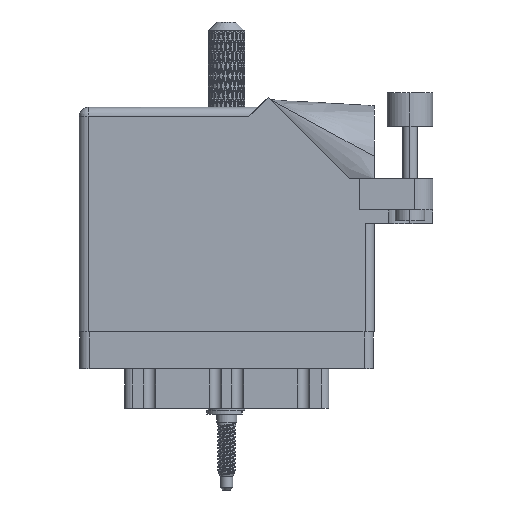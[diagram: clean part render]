
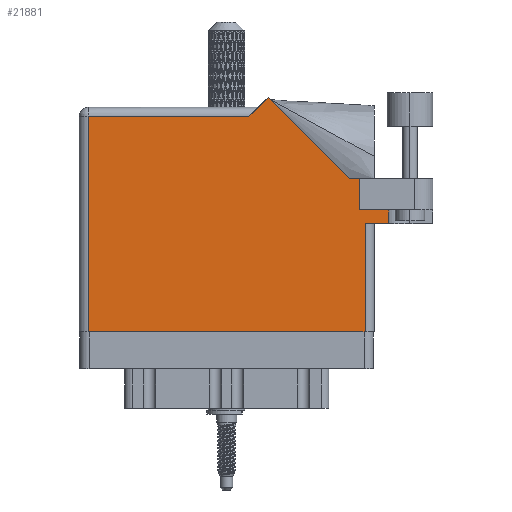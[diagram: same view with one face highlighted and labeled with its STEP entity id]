
A CAD part, front view. The second image highlights one B-rep face of the part: STEP entity #21881.
In plain terms, the highlighted face is planar.
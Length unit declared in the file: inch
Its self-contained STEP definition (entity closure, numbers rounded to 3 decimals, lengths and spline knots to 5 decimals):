
#1351 = EDGE_CURVE ( 'NONE', #46927, #65211, #44164, .T. ) ;
#1875 = VECTOR ( 'NONE', #19113, 39.37008 ) ;
#2982 = CARTESIAN_POINT ( 'NONE',  ( 1.28771, 1.60071, 0. ) ) ;
#3414 = EDGE_LOOP ( 'NONE', ( #64431, #32569, #68061, #83968, #47635, #10226, #4065, #5645, #94871, #12077, #34777 ) ) ;
#4065 = ORIENTED_EDGE ( 'NONE', *, *, #64842, .T. ) ;
#5645 = ORIENTED_EDGE ( 'NONE', *, *, #1351, .T. ) ;
#7933 = CARTESIAN_POINT ( 'NONE',  ( 2.1115, 0.737, 0. ) ) ;
#10226 = ORIENTED_EDGE ( 'NONE', *, *, #88782, .T. ) ;
#11178 = CARTESIAN_POINT ( 'NONE',  ( 1.91, 0.831, 0. ) ) ;
#12077 = ORIENTED_EDGE ( 'NONE', *, *, #70490, .T. ) ;
#12304 = VERTEX_POINT ( 'NONE', #50755 ) ;
#13783 = EDGE_CURVE ( 'NONE', #12304, #98223, #96820, .T. ) ;
#14642 = VECTOR ( 'NONE', #85014, 39.37008 ) ;
#17696 = EDGE_CURVE ( 'NONE', #98223, #33004, #19622, .T. ) ;
#19105 = VECTOR ( 'NONE', #43100, 39.37008 ) ;
#19113 = DIRECTION ( 'NONE',  ( 0., 1., 0. ) ) ;
#19622 = LINE ( 'NONE', #51916, #31186 ) ;
#19703 = CARTESIAN_POINT ( 'NONE',  ( 1.84442, 1.044, 0. ) ) ;
#20143 = DIRECTION ( 'NONE',  ( 0., -1., 0. ) ) ;
#20604 = CARTESIAN_POINT ( 'NONE',  ( 0.062, 0., 0. ) ) ;
#21535 = DIRECTION ( 'NONE',  ( -1., 0., 0. ) ) ;
#21881 = ADVANCED_FACE ( 'NONE', ( #37422 ), #69792, .F. ) ;
#24416 = VERTEX_POINT ( 'NONE', #57807 ) ;
#27063 = CARTESIAN_POINT ( 'NONE',  ( 0.062, 1.468, 0. ) ) ;
#29974 = DIRECTION ( 'NONE',  ( 0., 0., -1. ) ) ;
#31186 = VECTOR ( 'NONE', #20143, 39.37008 ) ;
#32569 = ORIENTED_EDGE ( 'NONE', *, *, #78292, .T. ) ;
#33004 = VERTEX_POINT ( 'NONE', #7933 ) ;
#33863 = VERTEX_POINT ( 'NONE', #51562 ) ;
#34357 = EDGE_CURVE ( 'NONE', #48647, #24416, #101630, .T. ) ;
#34777 = ORIENTED_EDGE ( 'NONE', *, *, #75810, .T. ) ;
#35055 = VECTOR ( 'NONE', #21535, 39.37008 ) ;
#36247 = CARTESIAN_POINT ( 'NONE',  ( 1.84442, 1.044, 0. ) ) ;
#37336 = AXIS2_PLACEMENT_3D ( 'NONE', #70317, #29974, #94724 ) ;
#37422 = FACE_OUTER_BOUND ( 'NONE', #3414, .T. ) ;
#40567 = VECTOR ( 'NONE', #48466, 39.37008 ) ;
#41432 = CARTESIAN_POINT ( 'NONE',  ( 2.01, 0.737, 0. ) ) ;
#43100 = DIRECTION ( 'NONE',  ( -0.707, 0.707, 0. ) ) ;
#43742 = CARTESIAN_POINT ( 'NONE',  ( 0., 0., 0. ) ) ;
#44164 = LINE ( 'NONE', #36247, #19105 ) ;
#45080 = DIRECTION ( 'NONE',  ( -0.707, -0.707, 0. ) ) ;
#46927 = VERTEX_POINT ( 'NONE', #19703 ) ;
#47635 = ORIENTED_EDGE ( 'NONE', *, *, #13783, .F. ) ;
#48466 = DIRECTION ( 'NONE',  ( 1., 0., 0. ) ) ;
#48647 = VERTEX_POINT ( 'NONE', #20604 ) ;
#48860 = DIRECTION ( 'NONE',  ( 1., 0., 0. ) ) ;
#49575 = CARTESIAN_POINT ( 'NONE',  ( 1.91, 1.044, 0. ) ) ;
#50669 = EDGE_CURVE ( 'NONE', #65211, #96211, #70080, .T. ) ;
#50755 = CARTESIAN_POINT ( 'NONE',  ( 1.91, 0.831, 0. ) ) ;
#51562 = CARTESIAN_POINT ( 'NONE',  ( 1.948, 0.737, 0. ) ) ;
#51916 = CARTESIAN_POINT ( 'NONE',  ( 2.1115, 1.16177, 0. ) ) ;
#53739 = DIRECTION ( 'NONE',  ( 0., 1., 0. ) ) ;
#54632 = CARTESIAN_POINT ( 'NONE',  ( 1.217, 1.53, 0. ) ) ;
#56406 = VECTOR ( 'NONE', #76155, 39.37008 ) ;
#56894 = VECTOR ( 'NONE', #82562, 39.37008 ) ;
#57807 = CARTESIAN_POINT ( 'NONE',  ( 1.948, 0., 0. ) ) ;
#58692 = VECTOR ( 'NONE', #53739, 39.37008 ) ;
#59422 = VECTOR ( 'NONE', #48860, 39.37008 ) ;
#59545 = LINE ( 'NONE', #86045, #14642 ) ;
#61194 = CARTESIAN_POINT ( 'NONE',  ( 1.948, 0.737, 0. ) ) ;
#61818 = LINE ( 'NONE', #94199, #35055 ) ;
#63855 = VERTEX_POINT ( 'NONE', #27063 ) ;
#64431 = ORIENTED_EDGE ( 'NONE', *, *, #34357, .T. ) ;
#64842 = EDGE_CURVE ( 'NONE', #103324, #46927, #59545, .T. ) ;
#65211 = VERTEX_POINT ( 'NONE', #2982 ) ;
#67151 = CARTESIAN_POINT ( 'NONE',  ( 2.1115, 0.831, 0. ) ) ;
#68061 = ORIENTED_EDGE ( 'NONE', *, *, #93259, .T. ) ;
#69172 = LINE ( 'NONE', #61194, #58692 ) ;
#69194 = VECTOR ( 'NONE', #45080, 39.37008 ) ;
#69792 = PLANE ( 'NONE',  #37336 ) ;
#70080 = LINE ( 'NONE', #54632, #69194 ) ;
#70317 = CARTESIAN_POINT ( 'NONE',  ( 0., 1.53, 0. ) ) ;
#70490 = EDGE_CURVE ( 'NONE', #96211, #63855, #61818, .T. ) ;
#71754 = LINE ( 'NONE', #41432, #59422 ) ;
#75810 = EDGE_CURVE ( 'NONE', #63855, #48647, #76179, .T. ) ;
#75852 = LINE ( 'NONE', #11178, #1875 ) ;
#76155 = DIRECTION ( 'NONE',  ( 1., 0., 0. ) ) ;
#76179 = LINE ( 'NONE', #83098, #56894 ) ;
#78292 = EDGE_CURVE ( 'NONE', #24416, #33863, #69172, .T. ) ;
#82562 = DIRECTION ( 'NONE',  ( 0., -1., 0. ) ) ;
#83098 = CARTESIAN_POINT ( 'NONE',  ( 0.062, 0., 0. ) ) ;
#83968 = ORIENTED_EDGE ( 'NONE', *, *, #17696, .F. ) ;
#85014 = DIRECTION ( 'NONE',  ( -1., 0., 0. ) ) ;
#86045 = CARTESIAN_POINT ( 'NONE',  ( 2.41, 1.044, 0. ) ) ;
#88782 = EDGE_CURVE ( 'NONE', #12304, #103324, #75852, .T. ) ;
#93259 = EDGE_CURVE ( 'NONE', #33863, #33004, #71754, .T. ) ;
#94199 = CARTESIAN_POINT ( 'NONE',  ( 0., 1.468, 0. ) ) ;
#94724 = DIRECTION ( 'NONE',  ( -1., 0., 0. ) ) ;
#94871 = ORIENTED_EDGE ( 'NONE', *, *, #50669, .T. ) ;
#96211 = VERTEX_POINT ( 'NONE', #100013 ) ;
#96820 = LINE ( 'NONE', #103215, #40567 ) ;
#98223 = VERTEX_POINT ( 'NONE', #67151 ) ;
#100013 = CARTESIAN_POINT ( 'NONE',  ( 1.155, 1.468, 0. ) ) ;
#101630 = LINE ( 'NONE', #43742, #56406 ) ;
#103215 = CARTESIAN_POINT ( 'NONE',  ( 1.91, 0.831, 0. ) ) ;
#103324 = VERTEX_POINT ( 'NONE', #49575 ) ;
